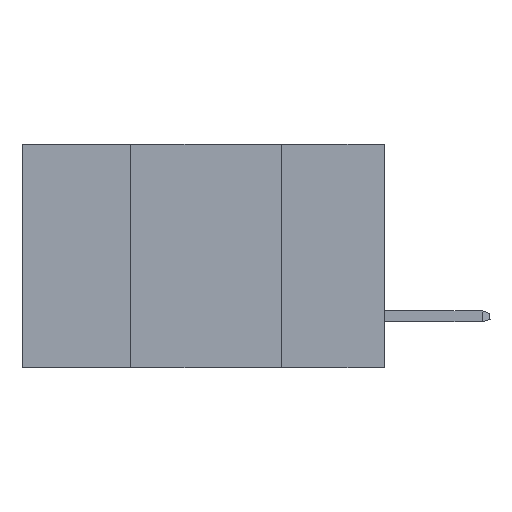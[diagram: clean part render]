
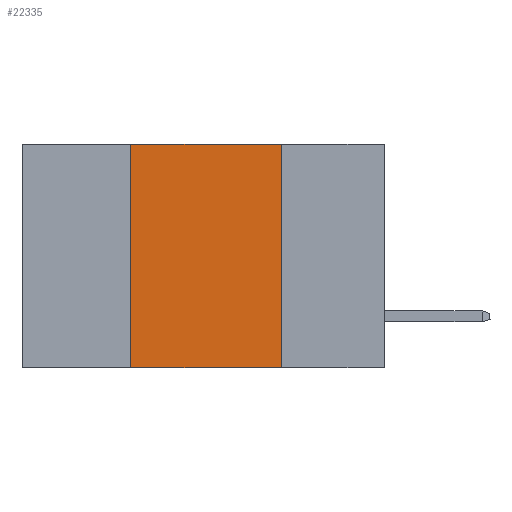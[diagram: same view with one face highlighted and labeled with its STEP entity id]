
A CAD part, left-side view. The second image highlights one B-rep face of the part: STEP entity #22335.
In plain terms, the highlighted planar face has unit normal (-1, 0, 0).
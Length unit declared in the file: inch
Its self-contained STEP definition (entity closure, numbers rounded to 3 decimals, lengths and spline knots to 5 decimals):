
#1 = LINE ( 'NONE', #13198, #857 ) ;
#685 = LINE ( 'NONE', #19881, #19563 ) ;
#857 = VECTOR ( 'NONE', #14991, 39.37008 ) ;
#1138 = VERTEX_POINT ( 'NONE', #22697 ) ;
#1351 = VERTEX_POINT ( 'NONE', #8504 ) ;
#2498 = ORIENTED_EDGE ( 'NONE', *, *, #12795, .F. ) ;
#2869 = ORIENTED_EDGE ( 'NONE', *, *, #17655, .F. ) ;
#3557 = VECTOR ( 'NONE', #7610, 39.37008 ) ;
#4251 = EDGE_CURVE ( 'NONE', #9726, #21786, #22422, .T. ) ;
#5999 = CARTESIAN_POINT ( 'NONE',  ( 0., 0.42, 0. ) ) ;
#6533 = FACE_OUTER_BOUND ( 'NONE', #13329, .T. ) ;
#7610 = DIRECTION ( 'NONE',  ( 0., -1., 0. ) ) ;
#8504 = CARTESIAN_POINT ( 'NONE',  ( 0., 0.17, -0.37 ) ) ;
#9726 = VERTEX_POINT ( 'NONE', #5999 ) ;
#10051 = CARTESIAN_POINT ( 'NONE',  ( 0., 0.17, 0. ) ) ;
#10757 = EDGE_CURVE ( 'NONE', #1138, #1351, #1, .T. ) ;
#11544 = DIRECTION ( 'NONE',  ( 0., 0., -1. ) ) ;
#12795 = EDGE_CURVE ( 'NONE', #21786, #1351, #23546, .T. ) ;
#13190 = ORIENTED_EDGE ( 'NONE', *, *, #4251, .F. ) ;
#13198 = CARTESIAN_POINT ( 'NONE',  ( 0., 0.6, -0.37 ) ) ;
#13329 = EDGE_LOOP ( 'NONE', ( #2498, #13190, #2869, #19015 ) ) ;
#13700 = CARTESIAN_POINT ( 'NONE',  ( 0., 0.17, 0. ) ) ;
#13805 = PLANE ( 'NONE',  #21736 ) ;
#14991 = DIRECTION ( 'NONE',  ( 0., -1., 0. ) ) ;
#17524 = DIRECTION ( 'NONE',  ( 0., 0., -1. ) ) ;
#17655 = EDGE_CURVE ( 'NONE', #1138, #9726, #685, .T. ) ;
#18669 = DIRECTION ( 'NONE',  ( 0., 0., 1. ) ) ;
#19015 = ORIENTED_EDGE ( 'NONE', *, *, #10757, .T. ) ;
#19049 = CARTESIAN_POINT ( 'NONE',  ( 0., 0.6, 0. ) ) ;
#19491 = CARTESIAN_POINT ( 'NONE',  ( 0., 0.6, 0. ) ) ;
#19496 = VECTOR ( 'NONE', #11544, 39.37008 ) ;
#19563 = VECTOR ( 'NONE', #18669, 39.37008 ) ;
#19881 = CARTESIAN_POINT ( 'NONE',  ( 0., 0.42, 0. ) ) ;
#21185 = DIRECTION ( 'NONE',  ( 1., 0., 0. ) ) ;
#21736 = AXIS2_PLACEMENT_3D ( 'NONE', #19491, #21185, #17524 ) ;
#21786 = VERTEX_POINT ( 'NONE', #10051 ) ;
#22335 = ADVANCED_FACE ( 'NONE', ( #6533 ), #13805, .F. ) ;
#22422 = LINE ( 'NONE', #19049, #3557 ) ;
#22697 = CARTESIAN_POINT ( 'NONE',  ( 0., 0.42, -0.37 ) ) ;
#23546 = LINE ( 'NONE', #13700, #19496 ) ;
